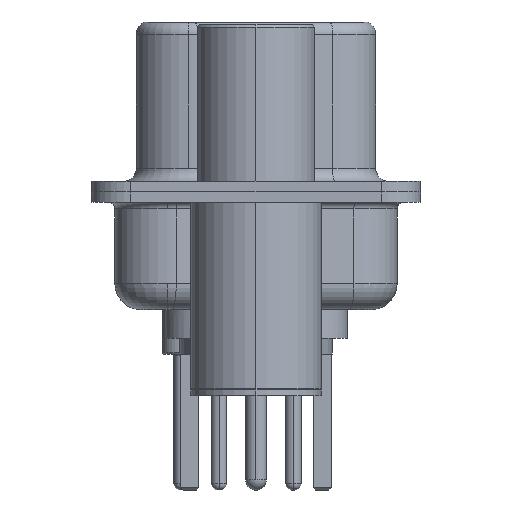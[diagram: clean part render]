
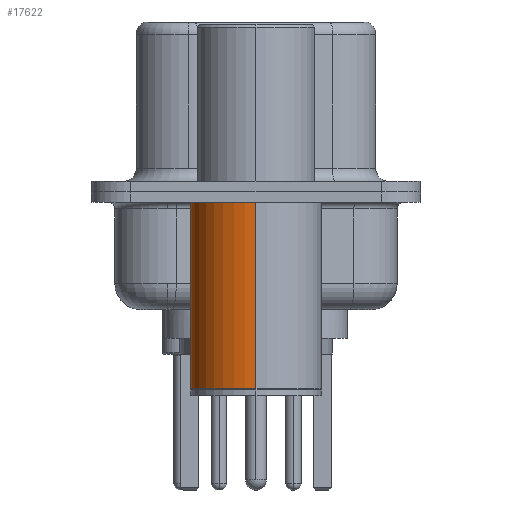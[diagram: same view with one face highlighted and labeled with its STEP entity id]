
A CAD part, left-side view. The second image highlights one B-rep face of the part: STEP entity #17622.
In plain terms, the highlighted cylindrical face has radius 2.5 mm (diameter 5 mm), a partial arc.
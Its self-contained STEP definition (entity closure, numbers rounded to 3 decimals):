
#630 = CARTESIAN_POINT ( 'NONE',  ( 2.5, 0., -7.525 ) ) ;
#840 = VERTEX_POINT ( 'NONE', #19776 ) ;
#1248 = LINE ( 'NONE', #7069, #22495 ) ;
#2861 = AXIS2_PLACEMENT_3D ( 'NONE', #21118, #7457, #23236 ) ;
#3503 = EDGE_CURVE ( 'NONE', #7961, #5704, #21540, .T. ) ;
#3693 = VECTOR ( 'NONE', #17633, 1000. ) ;
#3740 = DIRECTION ( 'NONE',  ( 0., 0., 1. ) ) ;
#5185 = CARTESIAN_POINT ( 'NONE',  ( 2.5, 0., -0.4 ) ) ;
#5704 = VERTEX_POINT ( 'NONE', #8932 ) ;
#7011 = EDGE_CURVE ( 'NONE', #14693, #840, #9115, .T. ) ;
#7022 = ORIENTED_EDGE ( 'NONE', *, *, #7011, .F. ) ;
#7069 = CARTESIAN_POINT ( 'NONE',  ( 2.5, 0., 0.581 ) ) ;
#7457 = DIRECTION ( 'NONE',  ( 0., 0., 1. ) ) ;
#7601 = EDGE_CURVE ( 'NONE', #7961, #14693, #1248, .T. ) ;
#7961 = VERTEX_POINT ( 'NONE', #630 ) ;
#8932 = CARTESIAN_POINT ( 'NONE',  ( -2.5, 0., -7.525 ) ) ;
#9115 = CIRCLE ( 'NONE', #20355, 2.5 ) ;
#11343 = CYLINDRICAL_SURFACE ( 'NONE', #2861, 2.5 ) ;
#11768 = ORIENTED_EDGE ( 'NONE', *, *, #3503, .T. ) ;
#12753 = EDGE_CURVE ( 'NONE', #5704, #840, #18255, .T. ) ;
#12919 = DIRECTION ( 'NONE',  ( 1., 0., 0. ) ) ;
#13752 = DIRECTION ( 'NONE',  ( 0., 0., 1. ) ) ;
#14001 = ORIENTED_EDGE ( 'NONE', *, *, #12753, .T. ) ;
#14022 = DIRECTION ( 'NONE',  ( 1., 0., 0. ) ) ;
#14693 = VERTEX_POINT ( 'NONE', #5185 ) ;
#15889 = CARTESIAN_POINT ( 'NONE',  ( 0., 0., -0.4 ) ) ;
#16811 = FACE_OUTER_BOUND ( 'NONE', #24098, .T. ) ;
#17622 = ADVANCED_FACE ( 'NONE', ( #16811 ), #11343, .T. ) ;
#17633 = DIRECTION ( 'NONE',  ( 0., 0., 1. ) ) ;
#17906 = ORIENTED_EDGE ( 'NONE', *, *, #7601, .F. ) ;
#18255 = LINE ( 'NONE', #20302, #3693 ) ;
#18864 = CARTESIAN_POINT ( 'NONE',  ( 0., 0., -7.525 ) ) ;
#19776 = CARTESIAN_POINT ( 'NONE',  ( -2.5, 0., -0.4 ) ) ;
#20302 = CARTESIAN_POINT ( 'NONE',  ( -2.5, 0., 0.581 ) ) ;
#20355 = AXIS2_PLACEMENT_3D ( 'NONE', #15889, #13752, #14022 ) ;
#20558 = DIRECTION ( 'NONE',  ( 0., 0., 1. ) ) ;
#21118 = CARTESIAN_POINT ( 'NONE',  ( 0., 0., 0.581 ) ) ;
#21540 = CIRCLE ( 'NONE', #23577, 2.5 ) ;
#22495 = VECTOR ( 'NONE', #3740, 1000. ) ;
#23236 = DIRECTION ( 'NONE',  ( 1., 0., 0. ) ) ;
#23577 = AXIS2_PLACEMENT_3D ( 'NONE', #18864, #20558, #12919 ) ;
#24098 = EDGE_LOOP ( 'NONE', ( #11768, #14001, #7022, #17906 ) ) ;
